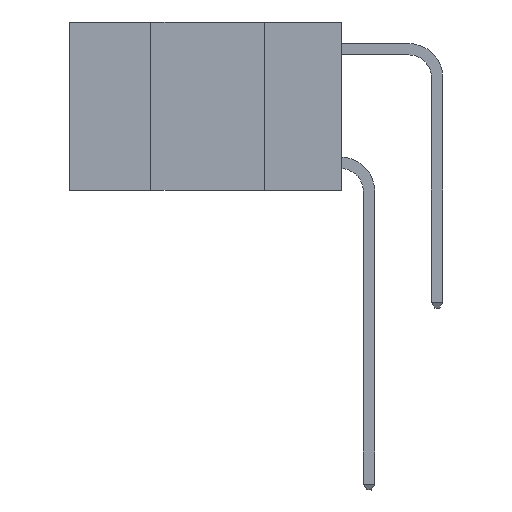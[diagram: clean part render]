
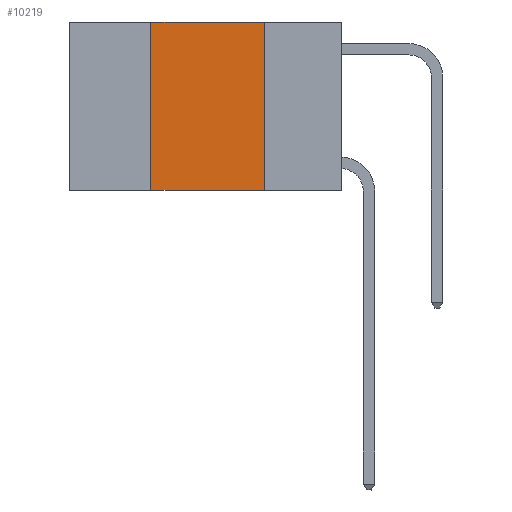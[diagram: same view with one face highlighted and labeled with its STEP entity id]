
A CAD part, left-side view. The second image highlights one B-rep face of the part: STEP entity #10219.
In plain terms, the highlighted planar face has unit normal (-1, 0, 0).
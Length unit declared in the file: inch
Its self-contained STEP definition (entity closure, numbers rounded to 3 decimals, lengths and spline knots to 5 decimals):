
#409 = AXIS2_PLACEMENT_3D ( 'NONE', #9443, #10532, #6399 ) ;
#733 = DIRECTION ( 'NONE',  ( 0., 0., 1. ) ) ;
#1551 = EDGE_CURVE ( 'NONE', #8192, #11638, #7590, .T. ) ;
#1604 = PLANE ( 'NONE',  #409 ) ;
#1783 = CARTESIAN_POINT ( 'NONE',  ( 0., 0.17, 0. ) ) ;
#2015 = CARTESIAN_POINT ( 'NONE',  ( 0., 0.42, 0. ) ) ;
#2717 = DIRECTION ( 'NONE',  ( 0., 0., -1. ) ) ;
#3452 = ORIENTED_EDGE ( 'NONE', *, *, #10372, .F. ) ;
#3620 = VECTOR ( 'NONE', #733, 39.37008 ) ;
#4052 = DIRECTION ( 'NONE',  ( 0., -1., 0. ) ) ;
#4072 = CARTESIAN_POINT ( 'NONE',  ( 0., 0.42, -0.37 ) ) ;
#4104 = DIRECTION ( 'NONE',  ( 0., -1., 0. ) ) ;
#4239 = EDGE_CURVE ( 'NONE', #5501, #12038, #12075, .T. ) ;
#4313 = VECTOR ( 'NONE', #4052, 39.37008 ) ;
#4415 = ORIENTED_EDGE ( 'NONE', *, *, #1551, .T. ) ;
#4744 = CARTESIAN_POINT ( 'NONE',  ( 0., 0.42, 0. ) ) ;
#4944 = VECTOR ( 'NONE', #4104, 39.37008 ) ;
#5025 = ORIENTED_EDGE ( 'NONE', *, *, #12537, .F. ) ;
#5088 = CARTESIAN_POINT ( 'NONE',  ( 0., 0.6, 0. ) ) ;
#5139 = EDGE_LOOP ( 'NONE', ( #5025, #10959, #3452, #4415 ) ) ;
#5501 = VERTEX_POINT ( 'NONE', #2015 ) ;
#6237 = LINE ( 'NONE', #4744, #3620 ) ;
#6399 = DIRECTION ( 'NONE',  ( 0., 0., -1. ) ) ;
#7590 = LINE ( 'NONE', #7854, #4944 ) ;
#7642 = CARTESIAN_POINT ( 'NONE',  ( 0., 0.17, 0. ) ) ;
#7854 = CARTESIAN_POINT ( 'NONE',  ( 0., 0.6, -0.37 ) ) ;
#8192 = VERTEX_POINT ( 'NONE', #4072 ) ;
#8309 = FACE_OUTER_BOUND ( 'NONE', #5139, .T. ) ;
#9166 = CARTESIAN_POINT ( 'NONE',  ( 0., 0.17, -0.37 ) ) ;
#9443 = CARTESIAN_POINT ( 'NONE',  ( 0., 0.6, 0. ) ) ;
#10219 = ADVANCED_FACE ( 'NONE', ( #8309 ), #1604, .F. ) ;
#10236 = LINE ( 'NONE', #7642, #12718 ) ;
#10372 = EDGE_CURVE ( 'NONE', #8192, #5501, #6237, .T. ) ;
#10532 = DIRECTION ( 'NONE',  ( 1., 0., 0. ) ) ;
#10959 = ORIENTED_EDGE ( 'NONE', *, *, #4239, .F. ) ;
#11638 = VERTEX_POINT ( 'NONE', #9166 ) ;
#12038 = VERTEX_POINT ( 'NONE', #1783 ) ;
#12075 = LINE ( 'NONE', #5088, #4313 ) ;
#12537 = EDGE_CURVE ( 'NONE', #12038, #11638, #10236, .T. ) ;
#12718 = VECTOR ( 'NONE', #2717, 39.37008 ) ;
